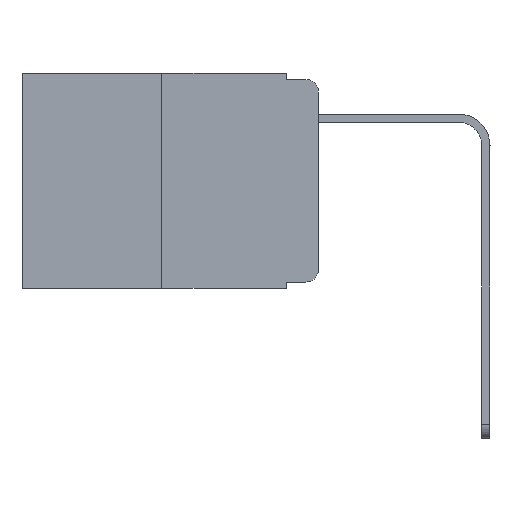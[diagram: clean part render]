
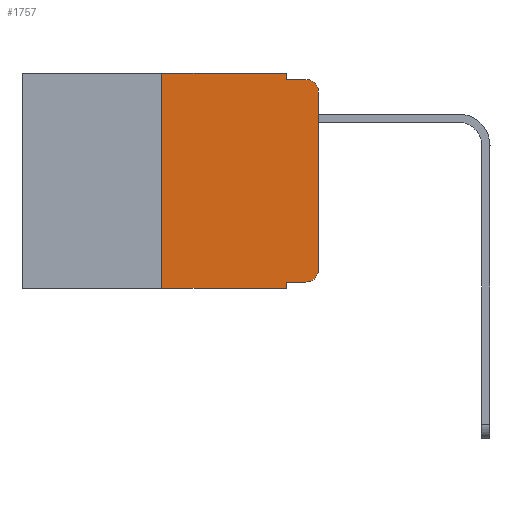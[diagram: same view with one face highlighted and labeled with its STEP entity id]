
A CAD part, left-side view. The second image highlights one B-rep face of the part: STEP entity #1757.
In plain terms, the highlighted planar face has unit normal (-1, 0, 0).
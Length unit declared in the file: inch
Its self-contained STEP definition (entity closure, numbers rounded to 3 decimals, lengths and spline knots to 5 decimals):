
#50 = VECTOR ( 'NONE', #10094, 39.37008 ) ;
#144 = DIRECTION ( 'NONE',  ( 0., -1., 0. ) ) ;
#344 = FACE_OUTER_BOUND ( 'NONE', #539, .T. ) ;
#539 = EDGE_LOOP ( 'NONE', ( #17357, #7389, #13919, #15301, #14056, #5740, #1234, #14546, #9058, #16785 ) ) ;
#711 = LINE ( 'NONE', #17429, #6674 ) ;
#737 = DIRECTION ( 'NONE',  ( 1., 0., 0. ) ) ;
#828 = DIRECTION ( 'NONE',  ( 0., 0., -1. ) ) ;
#1234 = ORIENTED_EDGE ( 'NONE', *, *, #8949, .T. ) ;
#1731 = CARTESIAN_POINT ( 'NONE',  ( 0., 0.02, -0.01 ) ) ;
#1757 = ADVANCED_FACE ( 'NONE', ( #344 ), #3338, .F. ) ;
#1904 = CARTESIAN_POINT ( 'NONE',  ( 0., 0., 0. ) ) ;
#1942 = VECTOR ( 'NONE', #828, 39.37008 ) ;
#2398 = VECTOR ( 'NONE', #3926, 39.37008 ) ;
#2406 = VECTOR ( 'NONE', #9511, 39.37008 ) ;
#2459 = CARTESIAN_POINT ( 'NONE',  ( 0., 0.051, -0.01 ) ) ;
#2821 = DIRECTION ( 'NONE',  ( -1., 0., 0. ) ) ;
#3187 = VERTEX_POINT ( 'NONE', #9427 ) ;
#3338 = PLANE ( 'NONE',  #17521 ) ;
#3556 = CARTESIAN_POINT ( 'NONE',  ( 0., 0.051, 0. ) ) ;
#3926 = DIRECTION ( 'NONE',  ( 0., 0., 1. ) ) ;
#4053 = CARTESIAN_POINT ( 'NONE',  ( 0., 0.473, 0. ) ) ;
#4197 = LINE ( 'NONE', #17126, #13237 ) ;
#4469 = LINE ( 'NONE', #3556, #1942 ) ;
#5011 = VERTEX_POINT ( 'NONE', #15771 ) ;
#5034 = DIRECTION ( 'NONE',  ( 0., 0., -1. ) ) ;
#5289 = CARTESIAN_POINT ( 'NONE',  ( 0., 0., -0.313 ) ) ;
#5451 = VERTEX_POINT ( 'NONE', #1731 ) ;
#5518 = EDGE_CURVE ( 'NONE', #16024, #8701, #4469, .T. ) ;
#5740 = ORIENTED_EDGE ( 'NONE', *, *, #7770, .F. ) ;
#6669 = DIRECTION ( 'NONE',  ( 0., -1., 0. ) ) ;
#6674 = VECTOR ( 'NONE', #13351, 39.37008 ) ;
#6712 = CARTESIAN_POINT ( 'NONE',  ( 0., 0.473, -0.343 ) ) ;
#7191 = VERTEX_POINT ( 'NONE', #14026 ) ;
#7307 = CARTESIAN_POINT ( 'NONE',  ( 0., 0.051, -0.343 ) ) ;
#7389 = ORIENTED_EDGE ( 'NONE', *, *, #15770, .T. ) ;
#7770 = EDGE_CURVE ( 'NONE', #7191, #9316, #14194, .T. ) ;
#8701 = VERTEX_POINT ( 'NONE', #7307 ) ;
#8949 = EDGE_CURVE ( 'NONE', #7191, #8701, #12655, .T. ) ;
#8977 = CARTESIAN_POINT ( 'NONE',  ( 0., 0.473, 0. ) ) ;
#9004 = VECTOR ( 'NONE', #144, 39.37008 ) ;
#9058 = ORIENTED_EDGE ( 'NONE', *, *, #10464, .T. ) ;
#9316 = VERTEX_POINT ( 'NONE', #14446 ) ;
#9427 = CARTESIAN_POINT ( 'NONE',  ( 0., 0.051, 0. ) ) ;
#9511 = DIRECTION ( 'NONE',  ( 0., -1., 0. ) ) ;
#9939 = CARTESIAN_POINT ( 'NONE',  ( 0., 0.051, -0.333 ) ) ;
#9979 = VERTEX_POINT ( 'NONE', #2459 ) ;
#10094 = DIRECTION ( 'NONE',  ( 0., 0., 1. ) ) ;
#10464 = EDGE_CURVE ( 'NONE', #16024, #16225, #4197, .T. ) ;
#10512 = CARTESIAN_POINT ( 'NONE',  ( 0., 0.051, -0.01 ) ) ;
#10699 = VERTEX_POINT ( 'NONE', #5289 ) ;
#11658 = LINE ( 'NONE', #10512, #12540 ) ;
#12092 = CARTESIAN_POINT ( 'NONE',  ( 0., 0.25, 0. ) ) ;
#12540 = VECTOR ( 'NONE', #6669, 39.37008 ) ;
#12655 = LINE ( 'NONE', #6712, #9004 ) ;
#12764 = DIRECTION ( 'NONE',  ( 0., -1., 0. ) ) ;
#13010 = DIRECTION ( 'NONE',  ( 0., 0., -1. ) ) ;
#13129 = LINE ( 'NONE', #1904, #50 ) ;
#13137 = LINE ( 'NONE', #4053, #2406 ) ;
#13237 = VECTOR ( 'NONE', #12764, 39.37008 ) ;
#13351 = DIRECTION ( 'NONE',  ( 0., 0., -1. ) ) ;
#13515 = EDGE_CURVE ( 'NONE', #10699, #5011, #13129, .T. ) ;
#13623 = CARTESIAN_POINT ( 'NONE',  ( 0., 0.02, -0.03 ) ) ;
#13756 = EDGE_CURVE ( 'NONE', #9979, #5451, #11658, .T. ) ;
#13919 = ORIENTED_EDGE ( 'NONE', *, *, #13756, .F. ) ;
#14026 = CARTESIAN_POINT ( 'NONE',  ( 0., 0.25, -0.343 ) ) ;
#14056 = ORIENTED_EDGE ( 'NONE', *, *, #16305, .F. ) ;
#14194 = LINE ( 'NONE', #12092, #2398 ) ;
#14446 = CARTESIAN_POINT ( 'NONE',  ( 0., 0.25, 0. ) ) ;
#14448 = CIRCLE ( 'NONE', #15563, 0.02 ) ;
#14546 = ORIENTED_EDGE ( 'NONE', *, *, #5518, .F. ) ;
#14672 = CIRCLE ( 'NONE', #16254, 0.02 ) ;
#14806 = CARTESIAN_POINT ( 'NONE',  ( 0., 0.02, -0.333 ) ) ;
#15301 = ORIENTED_EDGE ( 'NONE', *, *, #16754, .F. ) ;
#15563 = AXIS2_PLACEMENT_3D ( 'NONE', #17624, #17401, #5034 ) ;
#15602 = EDGE_CURVE ( 'NONE', #16225, #10699, #14448, .T. ) ;
#15770 = EDGE_CURVE ( 'NONE', #5011, #5451, #14672, .T. ) ;
#15771 = CARTESIAN_POINT ( 'NONE',  ( 0., 0., -0.03 ) ) ;
#16024 = VERTEX_POINT ( 'NONE', #9939 ) ;
#16225 = VERTEX_POINT ( 'NONE', #14806 ) ;
#16254 = AXIS2_PLACEMENT_3D ( 'NONE', #13623, #2821, #16380 ) ;
#16305 = EDGE_CURVE ( 'NONE', #9316, #3187, #13137, .T. ) ;
#16380 = DIRECTION ( 'NONE',  ( 0., 0., -1. ) ) ;
#16754 = EDGE_CURVE ( 'NONE', #3187, #9979, #711, .T. ) ;
#16785 = ORIENTED_EDGE ( 'NONE', *, *, #15602, .T. ) ;
#17126 = CARTESIAN_POINT ( 'NONE',  ( 0., 0.051, -0.333 ) ) ;
#17357 = ORIENTED_EDGE ( 'NONE', *, *, #13515, .T. ) ;
#17401 = DIRECTION ( 'NONE',  ( -1., 0., 0. ) ) ;
#17429 = CARTESIAN_POINT ( 'NONE',  ( 0., 0.051, 0. ) ) ;
#17521 = AXIS2_PLACEMENT_3D ( 'NONE', #8977, #737, #13010 ) ;
#17624 = CARTESIAN_POINT ( 'NONE',  ( 0., 0.02, -0.313 ) ) ;
